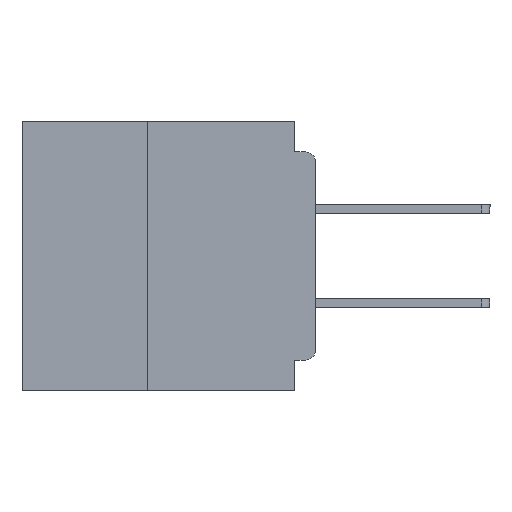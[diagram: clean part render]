
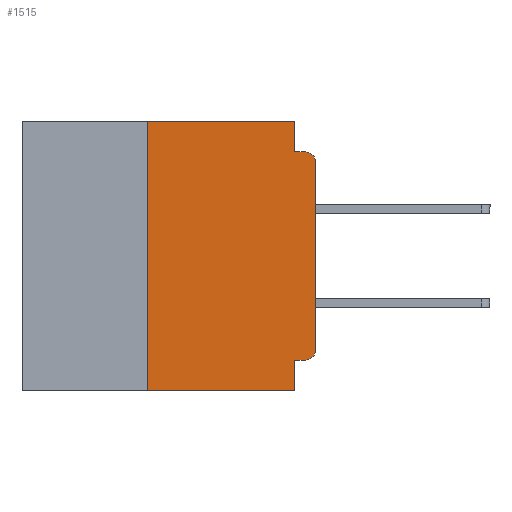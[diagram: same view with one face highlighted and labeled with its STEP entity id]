
A CAD part, left-side view. The second image highlights one B-rep face of the part: STEP entity #1515.
In plain terms, the highlighted planar face has unit normal (-1, 0, 0).
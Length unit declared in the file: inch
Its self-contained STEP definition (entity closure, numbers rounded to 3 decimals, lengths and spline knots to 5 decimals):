
#656 = CARTESIAN_POINT ( 'NONE',  ( 0., 0.25, -0.4 ) ) ;
#1022 = ORIENTED_EDGE ( 'NONE', *, *, #11999, .F. ) ;
#1097 = VERTEX_POINT ( 'NONE', #9399 ) ;
#1515 = ADVANCED_FACE ( 'NONE', ( #4009 ), #40068, .F. ) ;
#1915 = CARTESIAN_POINT ( 'NONE',  ( 0., 0.437, 0. ) ) ;
#2122 = DIRECTION ( 'NONE',  ( 0., -1., 0. ) ) ;
#2143 = VECTOR ( 'NONE', #2122, 39.37008 ) ;
#3391 = EDGE_CURVE ( 'NONE', #6116, #49318, #11886, .T. ) ;
#3418 = LINE ( 'NONE', #49151, #2143 ) ;
#4009 = FACE_OUTER_BOUND ( 'NONE', #50224, .T. ) ;
#4146 = LINE ( 'NONE', #656, #35514 ) ;
#5092 = LINE ( 'NONE', #43283, #45584 ) ;
#5955 = DIRECTION ( 'NONE',  ( 0., -1., 0. ) ) ;
#6116 = VERTEX_POINT ( 'NONE', #35346 ) ;
#6588 = CARTESIAN_POINT ( 'NONE',  ( 0., 0.015, -0.34 ) ) ;
#6729 = CARTESIAN_POINT ( 'NONE',  ( 0., 0.437, -0.4 ) ) ;
#7553 = CARTESIAN_POINT ( 'NONE',  ( 0., 0.437, 0. ) ) ;
#8961 = DIRECTION ( 'NONE',  ( -1., 0., 0. ) ) ;
#9399 = CARTESIAN_POINT ( 'NONE',  ( 0., 0.25, 0. ) ) ;
#10456 = ORIENTED_EDGE ( 'NONE', *, *, #24384, .T. ) ;
#10582 = DIRECTION ( 'NONE',  ( 0., 0., -1. ) ) ;
#10878 = CARTESIAN_POINT ( 'NONE',  ( 0., 0.031, -0.355 ) ) ;
#11886 = LINE ( 'NONE', #37241, #44330 ) ;
#11999 = EDGE_CURVE ( 'NONE', #38935, #48616, #3418, .T. ) ;
#12270 = VECTOR ( 'NONE', #23470, 39.37008 ) ;
#13011 = VECTOR ( 'NONE', #30504, 39.37008 ) ;
#13053 = AXIS2_PLACEMENT_3D ( 'NONE', #6588, #34096, #10582 ) ;
#13212 = AXIS2_PLACEMENT_3D ( 'NONE', #32496, #8961, #36387 ) ;
#13557 = EDGE_CURVE ( 'NONE', #21264, #38935, #43187, .T. ) ;
#14682 = LINE ( 'NONE', #1915, #23964 ) ;
#17039 = EDGE_CURVE ( 'NONE', #18004, #35734, #23516, .T. ) ;
#18004 = VERTEX_POINT ( 'NONE', #20511 ) ;
#19922 = DIRECTION ( 'NONE',  ( 0., 0., -1. ) ) ;
#20511 = CARTESIAN_POINT ( 'NONE',  ( 0., 0.25, -0.4 ) ) ;
#21264 = VERTEX_POINT ( 'NONE', #46935 ) ;
#21850 = EDGE_CURVE ( 'NONE', #48388, #35734, #5092, .T. ) ;
#23162 = CARTESIAN_POINT ( 'NONE',  ( 0., 0.015, -0.355 ) ) ;
#23470 = DIRECTION ( 'NONE',  ( 0., 1., 0. ) ) ;
#23516 = LINE ( 'NONE', #6729, #13011 ) ;
#23601 = ORIENTED_EDGE ( 'NONE', *, *, #34972, .F. ) ;
#23964 = VECTOR ( 'NONE', #5955, 39.37008 ) ;
#24274 = CARTESIAN_POINT ( 'NONE',  ( 0., 0., -0.06 ) ) ;
#24384 = EDGE_CURVE ( 'NONE', #49318, #48616, #47970, .T. ) ;
#27110 = DIRECTION ( 'NONE',  ( 0., 0., -1. ) ) ;
#28395 = DIRECTION ( 'NONE',  ( 0., 0., 1. ) ) ;
#29429 = AXIS2_PLACEMENT_3D ( 'NONE', #7553, #50877, #50865 ) ;
#29765 = VERTEX_POINT ( 'NONE', #23162 ) ;
#30504 = DIRECTION ( 'NONE',  ( 0., -1., 0. ) ) ;
#31052 = ORIENTED_EDGE ( 'NONE', *, *, #3391, .T. ) ;
#31110 = ORIENTED_EDGE ( 'NONE', *, *, #49630, .T. ) ;
#31832 = ORIENTED_EDGE ( 'NONE', *, *, #35343, .F. ) ;
#31900 = CARTESIAN_POINT ( 'NONE',  ( 0., 0.031, -0.4 ) ) ;
#32496 = CARTESIAN_POINT ( 'NONE',  ( 0., 0.015, -0.06 ) ) ;
#33140 = LINE ( 'NONE', #50527, #12270 ) ;
#34096 = DIRECTION ( 'NONE',  ( -1., 0., 0. ) ) ;
#34733 = CARTESIAN_POINT ( 'NONE',  ( 0., 0.031, 0. ) ) ;
#34972 = EDGE_CURVE ( 'NONE', #29765, #48388, #33140, .T. ) ;
#35064 = ORIENTED_EDGE ( 'NONE', *, *, #21850, .F. ) ;
#35343 = EDGE_CURVE ( 'NONE', #1097, #21264, #14682, .T. ) ;
#35346 = CARTESIAN_POINT ( 'NONE',  ( 0., 0., -0.34 ) ) ;
#35514 = VECTOR ( 'NONE', #28395, 39.37008 ) ;
#35714 = CARTESIAN_POINT ( 'NONE',  ( 0., 0.015, -0.045 ) ) ;
#35734 = VERTEX_POINT ( 'NONE', #31900 ) ;
#36387 = DIRECTION ( 'NONE',  ( 0., 0., -1. ) ) ;
#37241 = CARTESIAN_POINT ( 'NONE',  ( 0., 0., 0. ) ) ;
#37838 = DIRECTION ( 'NONE',  ( 0., 0., 1. ) ) ;
#38047 = ORIENTED_EDGE ( 'NONE', *, *, #49326, .F. ) ;
#38935 = VERTEX_POINT ( 'NONE', #47415 ) ;
#40068 = PLANE ( 'NONE',  #29429 ) ;
#40749 = VECTOR ( 'NONE', #27110, 39.37008 ) ;
#43187 = LINE ( 'NONE', #34733, #40749 ) ;
#43283 = CARTESIAN_POINT ( 'NONE',  ( 0., 0.031, -0.4 ) ) ;
#43393 = ORIENTED_EDGE ( 'NONE', *, *, #17039, .T. ) ;
#44330 = VECTOR ( 'NONE', #37838, 39.37008 ) ;
#45584 = VECTOR ( 'NONE', #19922, 39.37008 ) ;
#46935 = CARTESIAN_POINT ( 'NONE',  ( 0., 0.031, 0. ) ) ;
#47415 = CARTESIAN_POINT ( 'NONE',  ( 0., 0.031, -0.045 ) ) ;
#47970 = CIRCLE ( 'NONE', #13212, 0.015 ) ;
#48388 = VERTEX_POINT ( 'NONE', #10878 ) ;
#48616 = VERTEX_POINT ( 'NONE', #35714 ) ;
#49151 = CARTESIAN_POINT ( 'NONE',  ( 0., 0., -0.045 ) ) ;
#49318 = VERTEX_POINT ( 'NONE', #24274 ) ;
#49326 = EDGE_CURVE ( 'NONE', #18004, #1097, #4146, .T. ) ;
#49630 = EDGE_CURVE ( 'NONE', #29765, #6116, #50735, .T. ) ;
#50224 = EDGE_LOOP ( 'NONE', ( #31052, #10456, #1022, #50813, #31832, #38047, #43393, #35064, #23601, #31110 ) ) ;
#50527 = CARTESIAN_POINT ( 'NONE',  ( 0., 0., -0.355 ) ) ;
#50735 = CIRCLE ( 'NONE', #13053, 0.015 ) ;
#50813 = ORIENTED_EDGE ( 'NONE', *, *, #13557, .F. ) ;
#50865 = DIRECTION ( 'NONE',  ( 0., 0., -1. ) ) ;
#50877 = DIRECTION ( 'NONE',  ( 1., 0., 0. ) ) ;
